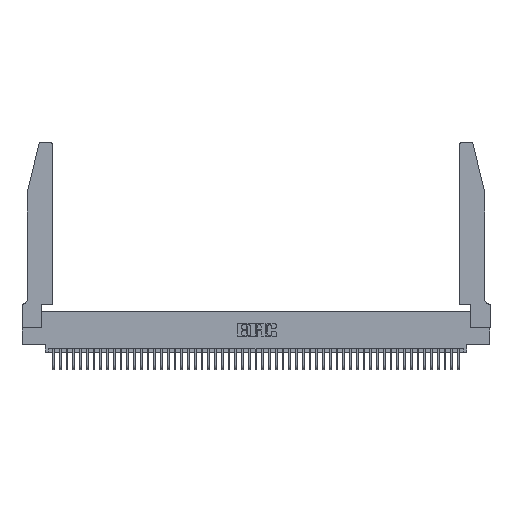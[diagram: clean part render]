
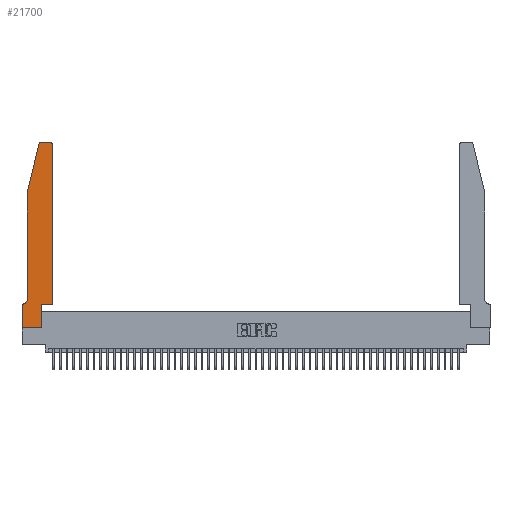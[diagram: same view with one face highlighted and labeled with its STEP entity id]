
A CAD part, top view. The second image highlights one B-rep face of the part: STEP entity #21700.
In plain terms, the highlighted planar face has unit normal (0, 0, 1).
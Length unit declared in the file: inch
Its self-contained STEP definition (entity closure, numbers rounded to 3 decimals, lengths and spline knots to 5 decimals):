
#180 = CARTESIAN_POINT ( 'NONE',  ( 0.0755, 0.35, 0.37 ) ) ;
#1501 = CARTESIAN_POINT ( 'NONE',  ( 0.0755, 2., 0.37 ) ) ;
#1628 = DIRECTION ( 'NONE',  ( 0., 0., 1. ) ) ;
#1745 = EDGE_CURVE ( 'NONE', #27332, #8929, #38995, .T. ) ;
#1799 = CARTESIAN_POINT ( 'NONE',  ( 0.2865, 0., 0.37 ) ) ;
#2141 = LINE ( 'NONE', #180, #20946 ) ;
#2414 = AXIS2_PLACEMENT_3D ( 'NONE', #41565, #19339, #45303 ) ;
#2781 = CARTESIAN_POINT ( 'NONE',  ( 0.4505, 0.35, 0.37 ) ) ;
#3533 = DIRECTION ( 'NONE',  ( 0., 1., 0. ) ) ;
#3631 = EDGE_CURVE ( 'NONE', #33526, #39800, #32608, .T. ) ;
#4293 = ORIENTED_EDGE ( 'NONE', *, *, #3631, .T. ) ;
#5167 = CARTESIAN_POINT ( 'NONE',  ( 0.4505, 0.35, 0.37 ) ) ;
#6173 = ORIENTED_EDGE ( 'NONE', *, *, #34339, .T. ) ;
#6369 = LINE ( 'NONE', #5167, #25114 ) ;
#6432 = EDGE_CURVE ( 'NONE', #22389, #22904, #39368, .T. ) ;
#6633 = VECTOR ( 'NONE', #23948, 39.37008 ) ;
#7477 = CARTESIAN_POINT ( 'NONE',  ( 0.0755, 2., 0.37 ) ) ;
#8899 = DIRECTION ( 'NONE',  ( 1., 0., 0. ) ) ;
#8929 = VERTEX_POINT ( 'NONE', #11011 ) ;
#10165 = CARTESIAN_POINT ( 'NONE',  ( 0.284, 2.75, 0.37 ) ) ;
#10569 = LINE ( 'NONE', #23794, #19391 ) ;
#10582 = EDGE_LOOP ( 'NONE', ( #25040, #6173, #4293, #34849, #33946, #15871, #10974, #36669, #23628, #41418, #43351, #31847 ) ) ;
#10974 = ORIENTED_EDGE ( 'NONE', *, *, #16117, .T. ) ;
#11011 = CARTESIAN_POINT ( 'NONE',  ( 0.0055, 0.35, 0.37 ) ) ;
#11716 = CARTESIAN_POINT ( 'NONE',  ( 0.4205, 2.75, 0.37 ) ) ;
#12532 = VERTEX_POINT ( 'NONE', #22840 ) ;
#13842 = CARTESIAN_POINT ( 'NONE',  ( 0.0755, 0.42, 0.37 ) ) ;
#14050 = VERTEX_POINT ( 'NONE', #2781 ) ;
#14832 = VECTOR ( 'NONE', #3533, 39.37008 ) ;
#15871 = ORIENTED_EDGE ( 'NONE', *, *, #41993, .T. ) ;
#16117 = EDGE_CURVE ( 'NONE', #30838, #12532, #46510, .T. ) ;
#16989 = CARTESIAN_POINT ( 'NONE',  ( 0., 0.35, 0.37 ) ) ;
#18546 = VERTEX_POINT ( 'NONE', #10165 ) ;
#18612 = DIRECTION ( 'NONE',  ( 0., -1., 0. ) ) ;
#18617 = CARTESIAN_POINT ( 'NONE',  ( 0., 0.35, 0.37 ) ) ;
#18853 = DIRECTION ( 'NONE',  ( -0.239, -0.971, 0. ) ) ;
#19339 = DIRECTION ( 'NONE',  ( 0., 0., -1. ) ) ;
#19391 = VECTOR ( 'NONE', #8899, 39.37008 ) ;
#19997 = CARTESIAN_POINT ( 'NONE',  ( 0.25487, 2.72718, 0.37 ) ) ;
#20393 = EDGE_CURVE ( 'NONE', #46453, #41538, #29275, .T. ) ;
#20746 = DIRECTION ( 'NONE',  ( 0., 0., 1. ) ) ;
#20892 = CARTESIAN_POINT ( 'NONE',  ( 0.284, 2.72, 0.37 ) ) ;
#20946 = VECTOR ( 'NONE', #44891, 39.37008 ) ;
#21615 = EDGE_CURVE ( 'NONE', #22904, #14050, #6369, .T. ) ;
#21700 = ADVANCED_FACE ( 'NONE', ( #22793 ), #42996, .T. ) ;
#22389 = VERTEX_POINT ( 'NONE', #1799 ) ;
#22793 = FACE_OUTER_BOUND ( 'NONE', #10582, .T. ) ;
#22840 = CARTESIAN_POINT ( 'NONE',  ( 0., 0., 0.37 ) ) ;
#22904 = VERTEX_POINT ( 'NONE', #27591 ) ;
#23628 = ORIENTED_EDGE ( 'NONE', *, *, #6432, .T. ) ;
#23794 = CARTESIAN_POINT ( 'NONE',  ( 0., 0., 0.37 ) ) ;
#23948 = DIRECTION ( 'NONE',  ( 0., -1., 0. ) ) ;
#24076 = CARTESIAN_POINT ( 'NONE',  ( 0.4205, 2.72, 0.37 ) ) ;
#24615 = DIRECTION ( 'NONE',  ( 1., 0., 0. ) ) ;
#25040 = ORIENTED_EDGE ( 'NONE', *, *, #27865, .T. ) ;
#25114 = VECTOR ( 'NONE', #38781, 39.37008 ) ;
#25188 = DIRECTION ( 'NONE',  ( -1., 0., 0. ) ) ;
#26007 = CARTESIAN_POINT ( 'NONE',  ( 0.0755, 2., 0.37 ) ) ;
#26557 = LINE ( 'NONE', #47419, #35300 ) ;
#26595 = DIRECTION ( 'NONE',  ( 0., 1., 0. ) ) ;
#26747 = VECTOR ( 'NONE', #18612, 39.37008 ) ;
#27332 = VERTEX_POINT ( 'NONE', #13842 ) ;
#27591 = CARTESIAN_POINT ( 'NONE',  ( 0.2865, 0.35, 0.37 ) ) ;
#27797 = DIRECTION ( 'NONE',  ( 1., 0., 0. ) ) ;
#27865 = EDGE_CURVE ( 'NONE', #41538, #18546, #26557, .T. ) ;
#28213 = CARTESIAN_POINT ( 'NONE',  ( 0.4505, 2.72, 0.37 ) ) ;
#28414 = AXIS2_PLACEMENT_3D ( 'NONE', #24076, #1628, #27797 ) ;
#28825 = EDGE_CURVE ( 'NONE', #39800, #27332, #34087, .T. ) ;
#29275 = CIRCLE ( 'NONE', #28414, 0.03 ) ;
#29443 = VECTOR ( 'NONE', #26595, 39.37008 ) ;
#30127 = EDGE_CURVE ( 'NONE', #14050, #46453, #44488, .T. ) ;
#30838 = VERTEX_POINT ( 'NONE', #18617 ) ;
#31847 = ORIENTED_EDGE ( 'NONE', *, *, #20393, .T. ) ;
#32608 = LINE ( 'NONE', #7477, #42501 ) ;
#33526 = VERTEX_POINT ( 'NONE', #19997 ) ;
#33568 = CIRCLE ( 'NONE', #46226, 0.03 ) ;
#33946 = ORIENTED_EDGE ( 'NONE', *, *, #1745, .T. ) ;
#34087 = LINE ( 'NONE', #1501, #6633 ) ;
#34339 = EDGE_CURVE ( 'NONE', #18546, #33526, #33568, .T. ) ;
#34849 = ORIENTED_EDGE ( 'NONE', *, *, #28825, .T. ) ;
#35300 = VECTOR ( 'NONE', #25188, 39.37008 ) ;
#36669 = ORIENTED_EDGE ( 'NONE', *, *, #36818, .T. ) ;
#36818 = EDGE_CURVE ( 'NONE', #12532, #22389, #10569, .T. ) ;
#37107 = CARTESIAN_POINT ( 'NONE',  ( 0., 0., 0.37 ) ) ;
#37684 = CARTESIAN_POINT ( 'NONE',  ( 0.2865, 0.35, 0.37 ) ) ;
#38781 = DIRECTION ( 'NONE',  ( 1., 0., 0. ) ) ;
#38995 = CIRCLE ( 'NONE', #2414, 0.07 ) ;
#39368 = LINE ( 'NONE', #37684, #29443 ) ;
#39800 = VERTEX_POINT ( 'NONE', #26007 ) ;
#41418 = ORIENTED_EDGE ( 'NONE', *, *, #21615, .T. ) ;
#41538 = VERTEX_POINT ( 'NONE', #11716 ) ;
#41565 = CARTESIAN_POINT ( 'NONE',  ( 0.0055, 0.42, 0.37 ) ) ;
#41993 = EDGE_CURVE ( 'NONE', #8929, #30838, #2141, .T. ) ;
#42501 = VECTOR ( 'NONE', #18853, 39.37008 ) ;
#42996 = PLANE ( 'NONE',  #44626 ) ;
#43351 = ORIENTED_EDGE ( 'NONE', *, *, #30127, .T. ) ;
#44488 = LINE ( 'NONE', #48159, #14832 ) ;
#44626 = AXIS2_PLACEMENT_3D ( 'NONE', #16989, #20746, #46702 ) ;
#44891 = DIRECTION ( 'NONE',  ( -1., 0., 0. ) ) ;
#45303 = DIRECTION ( 'NONE',  ( -1., 0., 0. ) ) ;
#46226 = AXIS2_PLACEMENT_3D ( 'NONE', #20892, #46848, #24615 ) ;
#46453 = VERTEX_POINT ( 'NONE', #28213 ) ;
#46510 = LINE ( 'NONE', #37107, #26747 ) ;
#46702 = DIRECTION ( 'NONE',  ( 1., 0., 0. ) ) ;
#46848 = DIRECTION ( 'NONE',  ( 0., 0., 1. ) ) ;
#47419 = CARTESIAN_POINT ( 'NONE',  ( 0.2605, 2.75, 0.37 ) ) ;
#48159 = CARTESIAN_POINT ( 'NONE',  ( 0.4505, 0.35, 0.37 ) ) ;
